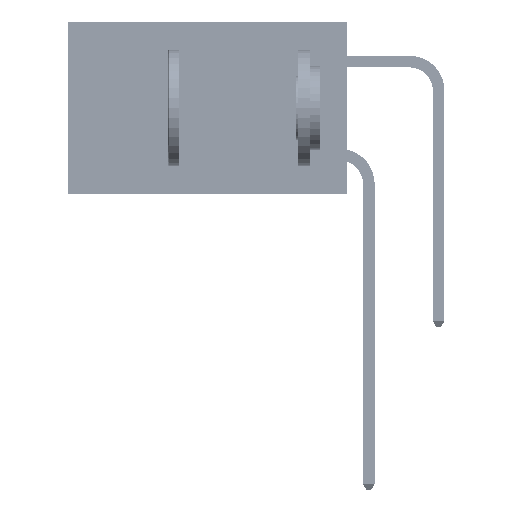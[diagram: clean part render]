
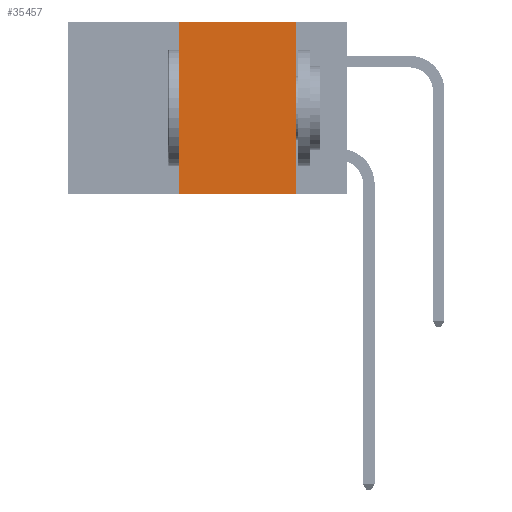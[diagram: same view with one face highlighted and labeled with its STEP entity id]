
A CAD part, left-side view. The second image highlights one B-rep face of the part: STEP entity #35457.
In plain terms, the highlighted planar face has unit normal (-1, 0, 0).
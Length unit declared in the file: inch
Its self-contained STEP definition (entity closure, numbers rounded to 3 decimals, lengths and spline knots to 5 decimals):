
#214 = ORIENTED_EDGE ( 'NONE', *, *, #32850, .F. ) ;
#320 = ORIENTED_EDGE ( 'NONE', *, *, #24990, .T. ) ;
#777 = CARTESIAN_POINT ( 'NONE',  ( 0., 0.36, 0. ) ) ;
#1573 = VECTOR ( 'NONE', #5555, 39.37008 ) ;
#3229 = VERTEX_POINT ( 'NONE', #32074 ) ;
#4258 = CARTESIAN_POINT ( 'NONE',  ( 0., 0.11, 0. ) ) ;
#5264 = CARTESIAN_POINT ( 'NONE',  ( 0., 0.6, -0.37 ) ) ;
#5555 = DIRECTION ( 'NONE',  ( 0., -1., 0. ) ) ;
#6326 = DIRECTION ( 'NONE',  ( 1., 0., 0. ) ) ;
#9018 = CARTESIAN_POINT ( 'NONE',  ( 0., 0.36, -0.37 ) ) ;
#10346 = CARTESIAN_POINT ( 'NONE',  ( 0., 0.6, 0. ) ) ;
#10590 = CARTESIAN_POINT ( 'NONE',  ( 0., 0.11, 0. ) ) ;
#11312 = LINE ( 'NONE', #5264, #47370 ) ;
#17111 = VERTEX_POINT ( 'NONE', #9018 ) ;
#19512 = VERTEX_POINT ( 'NONE', #4258 ) ;
#20013 = CARTESIAN_POINT ( 'NONE',  ( 0., 0.36, 0. ) ) ;
#21794 = LINE ( 'NONE', #10590, #45167 ) ;
#24822 = VERTEX_POINT ( 'NONE', #20013 ) ;
#24990 = EDGE_CURVE ( 'NONE', #17111, #3229, #11312, .T. ) ;
#25715 = VECTOR ( 'NONE', #39363, 39.37008 ) ;
#28013 = LINE ( 'NONE', #43845, #1573 ) ;
#29813 = EDGE_LOOP ( 'NONE', ( #214, #29871, #38517, #320 ) ) ;
#29871 = ORIENTED_EDGE ( 'NONE', *, *, #37737, .F. ) ;
#29884 = DIRECTION ( 'NONE',  ( 0., 0., -1. ) ) ;
#30694 = AXIS2_PLACEMENT_3D ( 'NONE', #10346, #6326, #33143 ) ;
#32074 = CARTESIAN_POINT ( 'NONE',  ( 0., 0.11, -0.37 ) ) ;
#32094 = DIRECTION ( 'NONE',  ( 0., -1., 0. ) ) ;
#32850 = EDGE_CURVE ( 'NONE', #19512, #3229, #21794, .T. ) ;
#33143 = DIRECTION ( 'NONE',  ( 0., 0., -1. ) ) ;
#34676 = LINE ( 'NONE', #777, #25715 ) ;
#35457 = ADVANCED_FACE ( 'NONE', ( #49279 ), #48798, .F. ) ;
#37737 = EDGE_CURVE ( 'NONE', #24822, #19512, #28013, .T. ) ;
#38517 = ORIENTED_EDGE ( 'NONE', *, *, #46201, .F. ) ;
#39363 = DIRECTION ( 'NONE',  ( 0., 0., 1. ) ) ;
#43845 = CARTESIAN_POINT ( 'NONE',  ( 0., 0.6, 0. ) ) ;
#45167 = VECTOR ( 'NONE', #29884, 39.37008 ) ;
#46201 = EDGE_CURVE ( 'NONE', #17111, #24822, #34676, .T. ) ;
#47370 = VECTOR ( 'NONE', #32094, 39.37008 ) ;
#48798 = PLANE ( 'NONE',  #30694 ) ;
#49279 = FACE_OUTER_BOUND ( 'NONE', #29813, .T. ) ;
